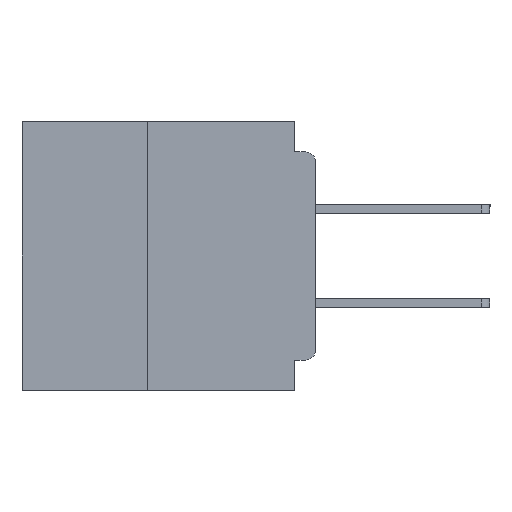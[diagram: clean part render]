
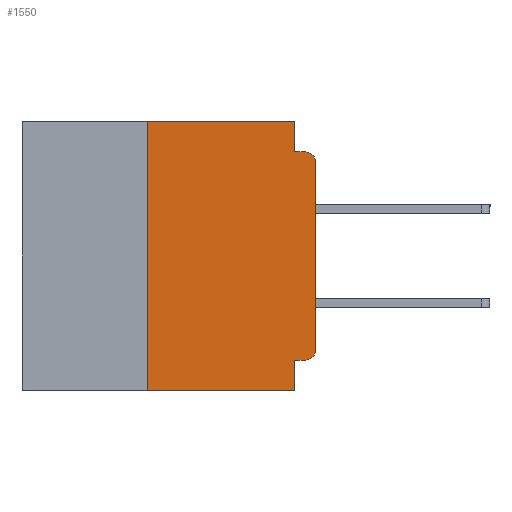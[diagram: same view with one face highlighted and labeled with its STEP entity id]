
A CAD part, left-side view. The second image highlights one B-rep face of the part: STEP entity #1550.
In plain terms, the highlighted planar face has unit normal (-1, 0, 0).
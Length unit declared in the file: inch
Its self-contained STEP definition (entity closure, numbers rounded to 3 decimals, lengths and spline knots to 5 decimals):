
#90 = DIRECTION ( 'NONE',  ( 0., 0., -1. ) ) ;
#227 = VERTEX_POINT ( 'NONE', #5766 ) ;
#1550 = ADVANCED_FACE ( 'NONE', ( #16955 ), #16351, .F. ) ;
#1796 = EDGE_CURVE ( 'NONE', #7571, #33270, #16495, .T. ) ;
#2084 = CARTESIAN_POINT ( 'NONE',  ( 0., 0.015, -0.06 ) ) ;
#2334 = DIRECTION ( 'NONE',  ( -1., 0., 0. ) ) ;
#2666 = CARTESIAN_POINT ( 'NONE',  ( 0., 0.25, -0.4 ) ) ;
#3335 = EDGE_CURVE ( 'NONE', #33270, #28672, #18175, .T. ) ;
#3721 = ORIENTED_EDGE ( 'NONE', *, *, #33991, .F. ) ;
#4116 = EDGE_CURVE ( 'NONE', #18354, #8586, #26289, .T. ) ;
#4393 = CARTESIAN_POINT ( 'NONE',  ( 0., 0., -0.06 ) ) ;
#4399 = DIRECTION ( 'NONE',  ( 0., 0., 1. ) ) ;
#4960 = DIRECTION ( 'NONE',  ( 0., 0., -1. ) ) ;
#5126 = LINE ( 'NONE', #18683, #26746 ) ;
#5217 = CARTESIAN_POINT ( 'NONE',  ( 0., 0.015, -0.355 ) ) ;
#5690 = CARTESIAN_POINT ( 'NONE',  ( 0., 0.437, 0. ) ) ;
#5766 = CARTESIAN_POINT ( 'NONE',  ( 0., 0.031, -0.355 ) ) ;
#7513 = EDGE_CURVE ( 'NONE', #26463, #18354, #36020, .T. ) ;
#7527 = VECTOR ( 'NONE', #28782, 39.37008 ) ;
#7571 = VERTEX_POINT ( 'NONE', #22378 ) ;
#7944 = CARTESIAN_POINT ( 'NONE',  ( 0., 0., -0.045 ) ) ;
#8043 = AXIS2_PLACEMENT_3D ( 'NONE', #2084, #22004, #4960 ) ;
#8445 = LINE ( 'NONE', #26054, #7527 ) ;
#8586 = VERTEX_POINT ( 'NONE', #4393 ) ;
#8721 = EDGE_CURVE ( 'NONE', #28672, #22829, #19373, .T. ) ;
#8991 = CARTESIAN_POINT ( 'NONE',  ( 0., 0., -0.34 ) ) ;
#12516 = VERTEX_POINT ( 'NONE', #31226 ) ;
#13163 = CIRCLE ( 'NONE', #8043, 0.015 ) ;
#13191 = CARTESIAN_POINT ( 'NONE',  ( 0., 0.437, 0. ) ) ;
#13934 = DIRECTION ( 'NONE',  ( 0., -1., 0. ) ) ;
#14259 = LINE ( 'NONE', #22899, #34497 ) ;
#14476 = ORIENTED_EDGE ( 'NONE', *, *, #4116, .T. ) ;
#14563 = DIRECTION ( 'NONE',  ( 1., 0., 0. ) ) ;
#16334 = ORIENTED_EDGE ( 'NONE', *, *, #3335, .F. ) ;
#16351 = PLANE ( 'NONE',  #27333 ) ;
#16482 = DIRECTION ( 'NONE',  ( 0., -1., 0. ) ) ;
#16495 = LINE ( 'NONE', #13191, #30265 ) ;
#16955 = FACE_OUTER_BOUND ( 'NONE', #24151, .T. ) ;
#17294 = VECTOR ( 'NONE', #24862, 39.37008 ) ;
#18022 = AXIS2_PLACEMENT_3D ( 'NONE', #19444, #2334, #22250 ) ;
#18081 = ORIENTED_EDGE ( 'NONE', *, *, #1796, .F. ) ;
#18175 = LINE ( 'NONE', #25483, #17294 ) ;
#18354 = VERTEX_POINT ( 'NONE', #8991 ) ;
#18683 = CARTESIAN_POINT ( 'NONE',  ( 0., 0.25, -0.4 ) ) ;
#18976 = EDGE_CURVE ( 'NONE', #8586, #22829, #13163, .T. ) ;
#18979 = VECTOR ( 'NONE', #28559, 39.37008 ) ;
#19373 = LINE ( 'NONE', #7944, #20244 ) ;
#19444 = CARTESIAN_POINT ( 'NONE',  ( 0., 0.015, -0.34 ) ) ;
#19637 = CARTESIAN_POINT ( 'NONE',  ( 0., 0.437, -0.4 ) ) ;
#19645 = VERTEX_POINT ( 'NONE', #2666 ) ;
#20244 = VECTOR ( 'NONE', #24799, 39.37008 ) ;
#20694 = ORIENTED_EDGE ( 'NONE', *, *, #28573, .F. ) ;
#21028 = CARTESIAN_POINT ( 'NONE',  ( 0., 0.031, 0. ) ) ;
#21388 = CARTESIAN_POINT ( 'NONE',  ( 0., 0.015, -0.045 ) ) ;
#22004 = DIRECTION ( 'NONE',  ( -1., 0., 0. ) ) ;
#22250 = DIRECTION ( 'NONE',  ( 0., 0., -1. ) ) ;
#22378 = CARTESIAN_POINT ( 'NONE',  ( 0., 0.25, 0. ) ) ;
#22451 = ORIENTED_EDGE ( 'NONE', *, *, #7513, .T. ) ;
#22829 = VERTEX_POINT ( 'NONE', #21388 ) ;
#22839 = ORIENTED_EDGE ( 'NONE', *, *, #8721, .F. ) ;
#22899 = CARTESIAN_POINT ( 'NONE',  ( 0., 0.031, -0.4 ) ) ;
#23756 = LINE ( 'NONE', #19637, #31019 ) ;
#24151 = EDGE_LOOP ( 'NONE', ( #14476, #29248, #22839, #16334, #18081, #3721, #27132, #20694, #35955, #22451 ) ) ;
#24799 = DIRECTION ( 'NONE',  ( 0., -1., 0. ) ) ;
#24862 = DIRECTION ( 'NONE',  ( 0., 0., -1. ) ) ;
#25483 = CARTESIAN_POINT ( 'NONE',  ( 0., 0.031, 0. ) ) ;
#26001 = CARTESIAN_POINT ( 'NONE',  ( 0., 0.031, -0.045 ) ) ;
#26054 = CARTESIAN_POINT ( 'NONE',  ( 0., 0., -0.355 ) ) ;
#26289 = LINE ( 'NONE', #28750, #18979 ) ;
#26338 = DIRECTION ( 'NONE',  ( 0., 0., -1. ) ) ;
#26463 = VERTEX_POINT ( 'NONE', #5217 ) ;
#26746 = VECTOR ( 'NONE', #4399, 39.37008 ) ;
#27132 = ORIENTED_EDGE ( 'NONE', *, *, #30433, .T. ) ;
#27333 = AXIS2_PLACEMENT_3D ( 'NONE', #5690, #14563, #26338 ) ;
#28559 = DIRECTION ( 'NONE',  ( 0., 0., 1. ) ) ;
#28573 = EDGE_CURVE ( 'NONE', #227, #12516, #14259, .T. ) ;
#28672 = VERTEX_POINT ( 'NONE', #26001 ) ;
#28750 = CARTESIAN_POINT ( 'NONE',  ( 0., 0., 0. ) ) ;
#28782 = DIRECTION ( 'NONE',  ( 0., 1., 0. ) ) ;
#29248 = ORIENTED_EDGE ( 'NONE', *, *, #18976, .T. ) ;
#30265 = VECTOR ( 'NONE', #16482, 39.37008 ) ;
#30433 = EDGE_CURVE ( 'NONE', #19645, #12516, #23756, .T. ) ;
#31019 = VECTOR ( 'NONE', #13934, 39.37008 ) ;
#31226 = CARTESIAN_POINT ( 'NONE',  ( 0., 0.031, -0.4 ) ) ;
#31806 = EDGE_CURVE ( 'NONE', #26463, #227, #8445, .T. ) ;
#33270 = VERTEX_POINT ( 'NONE', #21028 ) ;
#33991 = EDGE_CURVE ( 'NONE', #19645, #7571, #5126, .T. ) ;
#34497 = VECTOR ( 'NONE', #90, 39.37008 ) ;
#35955 = ORIENTED_EDGE ( 'NONE', *, *, #31806, .F. ) ;
#36020 = CIRCLE ( 'NONE', #18022, 0.015 ) ;
